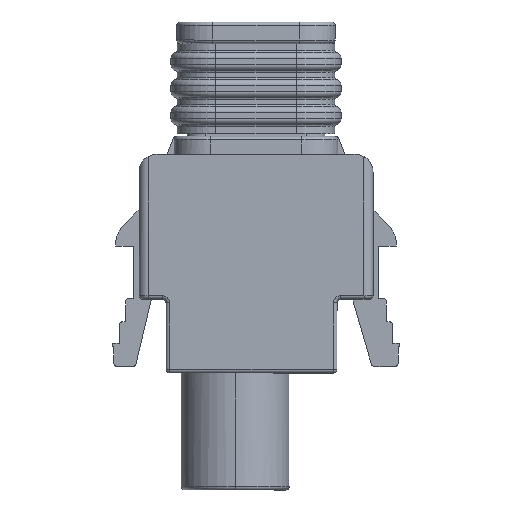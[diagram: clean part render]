
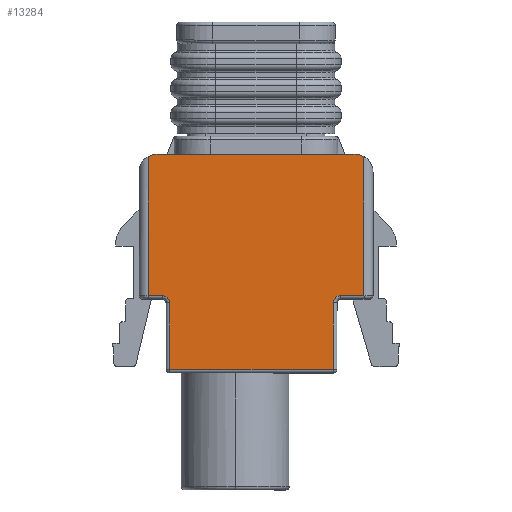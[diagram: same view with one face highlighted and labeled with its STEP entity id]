
A CAD part, left-side view. The second image highlights one B-rep face of the part: STEP entity #13284.
In plain terms, the highlighted planar face has unit normal (-1, 0, 0).
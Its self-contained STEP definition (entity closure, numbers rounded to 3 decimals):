
#501 = DIRECTION ( 'NONE',  ( 0., 0., 1. ) ) ;
#582 = DIRECTION ( 'NONE',  ( 0., -1., 0. ) ) ;
#636 = DIRECTION ( 'NONE',  ( 0., 1., 0. ) ) ;
#657 = CARTESIAN_POINT ( 'NONE',  ( -4.3, -4.3, -4.35 ) ) ;
#1120 = EDGE_CURVE ( 'NONE', #14751, #11690, #15367, .T. ) ;
#1150 = LINE ( 'NONE', #2638, #4628 ) ;
#1306 = EDGE_CURVE ( 'NONE', #6087, #14751, #10942, .T. ) ;
#1391 = CARTESIAN_POINT ( 'NONE',  ( -4.3, -6., -0.25 ) ) ;
#1399 = ORIENTED_EDGE ( 'NONE', *, *, #1120, .T. ) ;
#2145 = DIRECTION ( 'NONE',  ( 0., -0.5, 0.866 ) ) ;
#2158 = CARTESIAN_POINT ( 'NONE',  ( -4.3, -4.7, -0.25 ) ) ;
#2245 = CARTESIAN_POINT ( 'NONE',  ( -4.3, 6., -0.25 ) ) ;
#2327 = DIRECTION ( 'NONE',  ( -1., 0., 0. ) ) ;
#2388 = DIRECTION ( 'NONE',  ( 0., 0., 1. ) ) ;
#2449 = CARTESIAN_POINT ( 'NONE',  ( -4.3, -5.5, 7.6 ) ) ;
#2551 = DIRECTION ( 'NONE',  ( -1., 0., 0. ) ) ;
#2638 = CARTESIAN_POINT ( 'NONE',  ( -4.3, -6., -0.25 ) ) ;
#2679 = CARTESIAN_POINT ( 'NONE',  ( -4.3, 3.604, 7.6 ) ) ;
#2828 = EDGE_CURVE ( 'NONE', #15250, #16813, #15023, .T. ) ;
#2958 = ORIENTED_EDGE ( 'NONE', *, *, #14248, .T. ) ;
#3025 = ORIENTED_EDGE ( 'NONE', *, *, #3671, .T. ) ;
#3160 = AXIS2_PLACEMENT_3D ( 'NONE', #7084, #2551, #17014 ) ;
#3174 = CARTESIAN_POINT ( 'NONE',  ( -4.3, 6., -0.25 ) ) ;
#3521 = ORIENTED_EDGE ( 'NONE', *, *, #8306, .T. ) ;
#3660 = CARTESIAN_POINT ( 'NONE',  ( -4.3, 4.8, -0.65 ) ) ;
#3671 = EDGE_CURVE ( 'NONE', #16813, #16875, #16555, .T. ) ;
#3678 = VERTEX_POINT ( 'NONE', #18210 ) ;
#3693 = FACE_OUTER_BOUND ( 'NONE', #14306, .T. ) ;
#3716 = ORIENTED_EDGE ( 'NONE', *, *, #17711, .T. ) ;
#3782 = DIRECTION ( 'NONE',  ( 0., 1., 0. ) ) ;
#4352 = CARTESIAN_POINT ( 'NONE',  ( -4.3, 4.8, -4.35 ) ) ;
#4363 = EDGE_CURVE ( 'NONE', #15825, #3678, #8095, .T. ) ;
#4478 = VERTEX_POINT ( 'NONE', #1391 ) ;
#4628 = VECTOR ( 'NONE', #16917, 1000. ) ;
#4661 = VERTEX_POINT ( 'NONE', #2158 ) ;
#4728 = VERTEX_POINT ( 'NONE', #10092 ) ;
#4973 = CARTESIAN_POINT ( 'NONE',  ( -4.3, -4.3, -4.35 ) ) ;
#5315 = DIRECTION ( 'NONE',  ( 0., 1., 0. ) ) ;
#5574 = EDGE_CURVE ( 'NONE', #15133, #11690, #8992, .T. ) ;
#6022 = VECTOR ( 'NONE', #2388, 1000. ) ;
#6087 = VERTEX_POINT ( 'NONE', #8391 ) ;
#6680 = CARTESIAN_POINT ( 'NONE',  ( -4.3, -5.5, 6.6 ) ) ;
#6805 = AXIS2_PLACEMENT_3D ( 'NONE', #7964, #17702, #3782 ) ;
#7006 = AXIS2_PLACEMENT_3D ( 'NONE', #6680, #2327, #2145 ) ;
#7084 = CARTESIAN_POINT ( 'NONE',  ( -4.3, 5.5, 6.6 ) ) ;
#7203 = ORIENTED_EDGE ( 'NONE', *, *, #13307, .T. ) ;
#7639 = LINE ( 'NONE', #3174, #17500 ) ;
#7643 = LINE ( 'NONE', #11806, #12226 ) ;
#7689 = CARTESIAN_POINT ( 'NONE',  ( -4.3, 3.604, 7.6 ) ) ;
#7706 = VECTOR ( 'NONE', #8175, 1000. ) ;
#7964 = CARTESIAN_POINT ( 'NONE',  ( -4.3, -6.5, 7.6 ) ) ;
#8095 = LINE ( 'NONE', #2245, #7706 ) ;
#8175 = DIRECTION ( 'NONE',  ( 0., 0., 1. ) ) ;
#8218 = DIRECTION ( 'NONE',  ( 0., 0., -1. ) ) ;
#8306 = EDGE_CURVE ( 'NONE', #15825, #6087, #7639, .T. ) ;
#8391 = CARTESIAN_POINT ( 'NONE',  ( -4.3, 5.2, -0.25 ) ) ;
#8947 = VECTOR ( 'NONE', #16525, 1000. ) ;
#8992 = LINE ( 'NONE', #657, #8947 ) ;
#9288 = ORIENTED_EDGE ( 'NONE', *, *, #4363, .F. ) ;
#9431 = EDGE_CURVE ( 'NONE', #15262, #16875, #7643, .T. ) ;
#9696 = CARTESIAN_POINT ( 'NONE',  ( -4.3, 4.8, -0.65 ) ) ;
#9845 = ORIENTED_EDGE ( 'NONE', *, *, #18211, .T. ) ;
#10092 = CARTESIAN_POINT ( 'NONE',  ( -4.3, 5.5, 7.6 ) ) ;
#10126 = VERTEX_POINT ( 'NONE', #11314 ) ;
#10177 = CARTESIAN_POINT ( 'NONE',  ( -4.3, -6., 7.466 ) ) ;
#10243 = DIRECTION ( 'NONE',  ( 1., 0., 0. ) ) ;
#10528 = CARTESIAN_POINT ( 'NONE',  ( -4.3, 6., -0.25 ) ) ;
#10566 = CARTESIAN_POINT ( 'NONE',  ( -4.3, -4.7, -0.65 ) ) ;
#10622 = CARTESIAN_POINT ( 'NONE',  ( -4.3, -5.5, 7.6 ) ) ;
#10942 = CIRCLE ( 'NONE', #13318, 0.4 ) ;
#11314 = CARTESIAN_POINT ( 'NONE',  ( -4.3, -4.3, -0.65 ) ) ;
#11318 = LINE ( 'NONE', #15410, #12426 ) ;
#11359 = EDGE_CURVE ( 'NONE', #4728, #3678, #14730, .T. ) ;
#11369 = EDGE_CURVE ( 'NONE', #4478, #15250, #1150, .T. ) ;
#11690 = VERTEX_POINT ( 'NONE', #4352 ) ;
#11806 = CARTESIAN_POINT ( 'NONE',  ( -4.3, 3.604, 7.6 ) ) ;
#12047 = DIRECTION ( 'NONE',  ( 1., 0., 0. ) ) ;
#12226 = VECTOR ( 'NONE', #17746, 1000. ) ;
#12426 = VECTOR ( 'NONE', #13837, 1000. ) ;
#12571 = CARTESIAN_POINT ( 'NONE',  ( -4.3, -3.604, 7.6 ) ) ;
#13284 = ADVANCED_FACE ( 'NONE', ( #3693 ), #17892, .T. ) ;
#13307 = EDGE_CURVE ( 'NONE', #15262, #4728, #14748, .T. ) ;
#13318 = AXIS2_PLACEMENT_3D ( 'NONE', #17474, #10243, #501 ) ;
#13837 = DIRECTION ( 'NONE',  ( 0., -1., 0. ) ) ;
#13935 = VECTOR ( 'NONE', #636, 1000. ) ;
#14035 = ORIENTED_EDGE ( 'NONE', *, *, #11369, .T. ) ;
#14248 = EDGE_CURVE ( 'NONE', #4661, #4478, #11318, .T. ) ;
#14306 = EDGE_LOOP ( 'NONE', ( #15862, #3025, #15948, #7203, #14460, #9288, #3521, #17982, #1399, #17142, #3716, #9845, #2958, #14035 ) ) ;
#14460 = ORIENTED_EDGE ( 'NONE', *, *, #11359, .T. ) ;
#14730 = CIRCLE ( 'NONE', #3160, 1. ) ;
#14748 = LINE ( 'NONE', #7689, #13935 ) ;
#14751 = VERTEX_POINT ( 'NONE', #3660 ) ;
#14833 = LINE ( 'NONE', #4973, #6022 ) ;
#14944 = DIRECTION ( 'NONE',  ( 0., 1., 0. ) ) ;
#15023 = CIRCLE ( 'NONE', #7006, 1. ) ;
#15133 = VERTEX_POINT ( 'NONE', #17899 ) ;
#15250 = VERTEX_POINT ( 'NONE', #10177 ) ;
#15262 = VERTEX_POINT ( 'NONE', #2679 ) ;
#15367 = LINE ( 'NONE', #9696, #17854 ) ;
#15380 = AXIS2_PLACEMENT_3D ( 'NONE', #10566, #12047, #14944 ) ;
#15410 = CARTESIAN_POINT ( 'NONE',  ( -4.3, -4.7, -0.25 ) ) ;
#15788 = VECTOR ( 'NONE', #5315, 1000. ) ;
#15825 = VERTEX_POINT ( 'NONE', #10528 ) ;
#15862 = ORIENTED_EDGE ( 'NONE', *, *, #2828, .T. ) ;
#15948 = ORIENTED_EDGE ( 'NONE', *, *, #9431, .F. ) ;
#16525 = DIRECTION ( 'NONE',  ( 0., 1., 0. ) ) ;
#16555 = LINE ( 'NONE', #2449, #15788 ) ;
#16577 = CIRCLE ( 'NONE', #15380, 0.4 ) ;
#16813 = VERTEX_POINT ( 'NONE', #10622 ) ;
#16875 = VERTEX_POINT ( 'NONE', #12571 ) ;
#16917 = DIRECTION ( 'NONE',  ( 0., 0., 1. ) ) ;
#17014 = DIRECTION ( 'NONE',  ( 0., 0., 1. ) ) ;
#17142 = ORIENTED_EDGE ( 'NONE', *, *, #5574, .F. ) ;
#17474 = CARTESIAN_POINT ( 'NONE',  ( -4.3, 5.2, -0.65 ) ) ;
#17500 = VECTOR ( 'NONE', #582, 1000. ) ;
#17702 = DIRECTION ( 'NONE',  ( -1., 0., 0. ) ) ;
#17711 = EDGE_CURVE ( 'NONE', #15133, #10126, #14833, .T. ) ;
#17746 = DIRECTION ( 'NONE',  ( 0., -1., 0. ) ) ;
#17854 = VECTOR ( 'NONE', #8218, 1000. ) ;
#17892 = PLANE ( 'NONE',  #6805 ) ;
#17899 = CARTESIAN_POINT ( 'NONE',  ( -4.3, -4.3, -4.35 ) ) ;
#17982 = ORIENTED_EDGE ( 'NONE', *, *, #1306, .T. ) ;
#18210 = CARTESIAN_POINT ( 'NONE',  ( -4.3, 6., 7.466 ) ) ;
#18211 = EDGE_CURVE ( 'NONE', #10126, #4661, #16577, .T. ) ;
